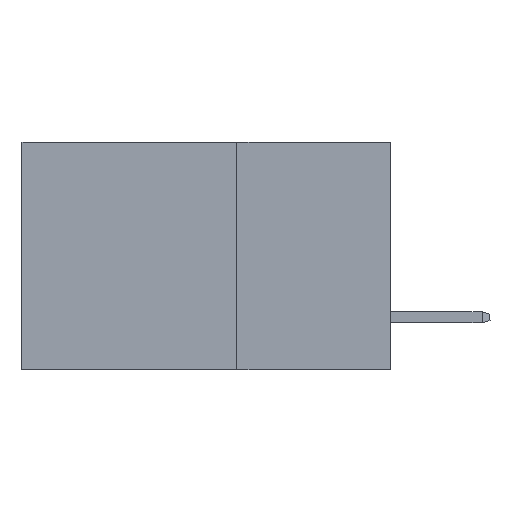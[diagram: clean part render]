
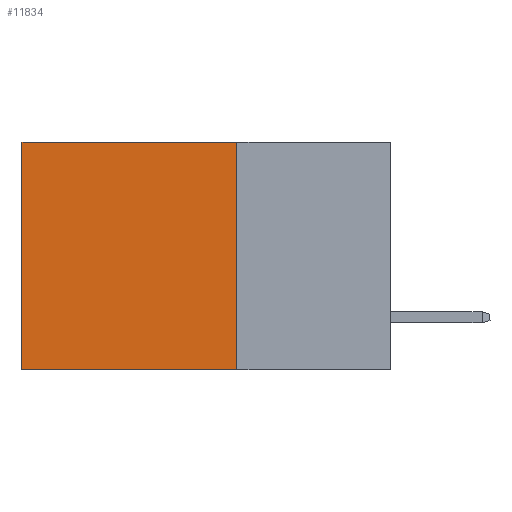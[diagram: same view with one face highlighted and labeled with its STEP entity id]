
A CAD part, left-side view. The second image highlights one B-rep face of the part: STEP entity #11834.
In plain terms, the highlighted planar face has unit normal (-1, 0, 0).
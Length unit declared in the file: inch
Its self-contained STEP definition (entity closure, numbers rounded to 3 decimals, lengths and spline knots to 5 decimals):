
#542 = ORIENTED_EDGE ( 'NONE', *, *, #581, .T. ) ;
#581 = EDGE_CURVE ( 'NONE', #1362, #9688, #3774, .T. ) ;
#696 = EDGE_CURVE ( 'NONE', #14580, #9688, #8664, .T. ) ;
#943 = DIRECTION ( 'NONE',  ( 0., 0., -1. ) ) ;
#1362 = VERTEX_POINT ( 'NONE', #13749 ) ;
#2068 = CARTESIAN_POINT ( 'NONE',  ( 0.2875, 0.6, 0. ) ) ;
#2098 = AXIS2_PLACEMENT_3D ( 'NONE', #9453, #15543, #943 ) ;
#2117 = EDGE_CURVE ( 'NONE', #4026, #14580, #7771, .T. ) ;
#3255 = DIRECTION ( 'NONE',  ( 0., 1., 0. ) ) ;
#3432 = LINE ( 'NONE', #4033, #4732 ) ;
#3774 = LINE ( 'NONE', #2068, #10554 ) ;
#4026 = VERTEX_POINT ( 'NONE', #8656 ) ;
#4033 = CARTESIAN_POINT ( 'NONE',  ( 0.2875, 0.25, 0. ) ) ;
#4409 = ORIENTED_EDGE ( 'NONE', *, *, #2117, .F. ) ;
#4506 = CARTESIAN_POINT ( 'NONE',  ( 0.2875, 0.6, -0.37 ) ) ;
#4732 = VECTOR ( 'NONE', #6843, 39.37008 ) ;
#6843 = DIRECTION ( 'NONE',  ( 0., 1., 0. ) ) ;
#7097 = PLANE ( 'NONE',  #2098 ) ;
#7771 = LINE ( 'NONE', #12515, #13740 ) ;
#8656 = CARTESIAN_POINT ( 'NONE',  ( 0.2875, 0.25, 0. ) ) ;
#8664 = LINE ( 'NONE', #9210, #11462 ) ;
#9002 = EDGE_LOOP ( 'NONE', ( #542, #13097, #4409, #14413 ) ) ;
#9210 = CARTESIAN_POINT ( 'NONE',  ( 0.2875, 0.25, -0.37 ) ) ;
#9453 = CARTESIAN_POINT ( 'NONE',  ( 0.2875, 0.25, 0. ) ) ;
#9688 = VERTEX_POINT ( 'NONE', #4506 ) ;
#10012 = CARTESIAN_POINT ( 'NONE',  ( 0.2875, 0.25, -0.37 ) ) ;
#10554 = VECTOR ( 'NONE', #11500, 39.37008 ) ;
#10639 = FACE_OUTER_BOUND ( 'NONE', #9002, .T. ) ;
#11462 = VECTOR ( 'NONE', #3255, 39.37008 ) ;
#11500 = DIRECTION ( 'NONE',  ( 0., 0., -1. ) ) ;
#11834 = ADVANCED_FACE ( 'NONE', ( #10639 ), #7097, .F. ) ;
#12515 = CARTESIAN_POINT ( 'NONE',  ( 0.2875, 0.25, 0. ) ) ;
#13097 = ORIENTED_EDGE ( 'NONE', *, *, #696, .F. ) ;
#13413 = EDGE_CURVE ( 'NONE', #4026, #1362, #3432, .T. ) ;
#13706 = DIRECTION ( 'NONE',  ( 0., 0., -1. ) ) ;
#13740 = VECTOR ( 'NONE', #13706, 39.37008 ) ;
#13749 = CARTESIAN_POINT ( 'NONE',  ( 0.2875, 0.6, 0. ) ) ;
#14413 = ORIENTED_EDGE ( 'NONE', *, *, #13413, .T. ) ;
#14580 = VERTEX_POINT ( 'NONE', #10012 ) ;
#15543 = DIRECTION ( 'NONE',  ( 1., 0., 0. ) ) ;
